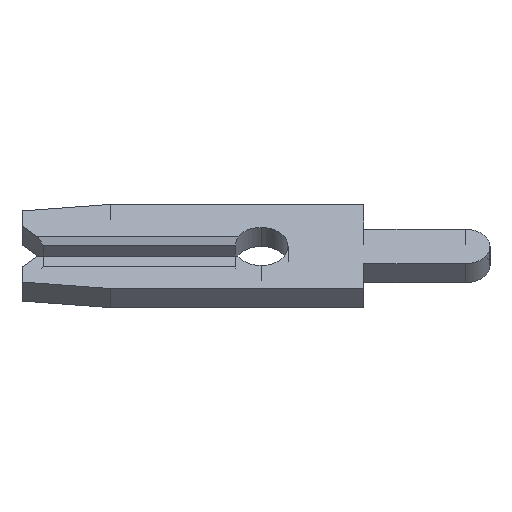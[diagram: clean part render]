
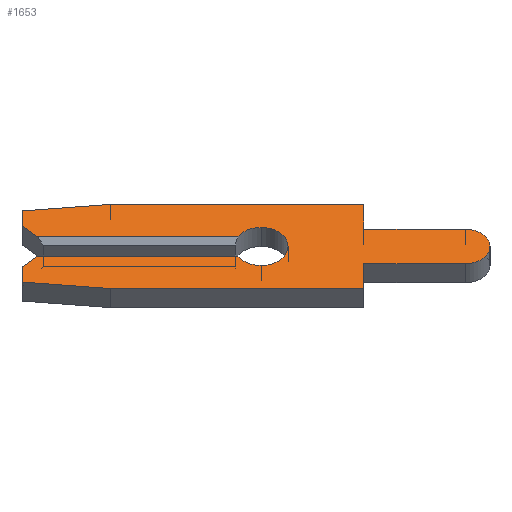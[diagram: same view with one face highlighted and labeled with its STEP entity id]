
A CAD part, left-side view. The second image highlights one B-rep face of the part: STEP entity #1653.
In plain terms, the highlighted face is planar.
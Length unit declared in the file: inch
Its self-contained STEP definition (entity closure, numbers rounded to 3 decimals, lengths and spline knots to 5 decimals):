
#2 = LINE ( 'NONE', #1609, #280 ) ;
#39 = EDGE_CURVE ( 'NONE', #1831, #1373, #1996, .T. ) ;
#45 = CARTESIAN_POINT ( 'NONE',  ( -0.013, 0., 0. ) ) ;
#47 = AXIS2_PLACEMENT_3D ( 'NONE', #45, #1066, #555 ) ;
#59 = VERTEX_POINT ( 'NONE', #773 ) ;
#92 = DIRECTION ( 'NONE',  ( 0., 0., -1. ) ) ;
#144 = AXIS2_PLACEMENT_3D ( 'NONE', #2043, #637, #298 ) ;
#159 = LINE ( 'NONE', #165, #1851 ) ;
#165 = CARTESIAN_POINT ( 'NONE',  ( -0.013, 0., -0.013 ) ) ;
#181 = VECTOR ( 'NONE', #1520, 39.37008 ) ;
#214 = AXIS2_PLACEMENT_3D ( 'NONE', #967, #972, #92 ) ;
#235 = EDGE_CURVE ( 'NONE', #1225, #517, #470, .T. ) ;
#260 = EDGE_CURVE ( 'NONE', #429, #533, #822, .T. ) ;
#280 = VECTOR ( 'NONE', #522, 39.37008 ) ;
#284 = CARTESIAN_POINT ( 'NONE',  ( -0.013, 0.2105, -0.0075 ) ) ;
#298 = DIRECTION ( 'NONE',  ( 0., 0., 1. ) ) ;
#301 = DIRECTION ( 'NONE',  ( 0., -1., 0. ) ) ;
#304 = VECTOR ( 'NONE', #2030, 39.37008 ) ;
#310 = ORIENTED_EDGE ( 'NONE', *, *, #260, .F. ) ;
#320 = CARTESIAN_POINT ( 'NONE',  ( -0.013, -0.099, -0.0235 ) ) ;
#329 = DIRECTION ( 'NONE',  ( -1., 0., 0. ) ) ;
#363 = EDGE_LOOP ( 'NONE', ( #1891, #2097, #483, #1398, #2093, #1008, #310, #1164, #1165, #1223, #1648, #1357, #1426, #921, #996, #947, #1850, #514 ) ) ;
#373 = CARTESIAN_POINT ( 'NONE',  ( -0.013, -0.099, 0.0235 ) ) ;
#401 = CARTESIAN_POINT ( 'NONE',  ( -0.013, -0.1975, -0.0235 ) ) ;
#408 = EDGE_CURVE ( 'NONE', #539, #59, #1124, .T. ) ;
#429 = VERTEX_POINT ( 'NONE', #2178 ) ;
#450 = DIRECTION ( 'NONE',  ( 0., 0.707, 0.707 ) ) ;
#460 = CARTESIAN_POINT ( 'NONE',  ( -0.013, -0.099, 0.0575 ) ) ;
#470 = LINE ( 'NONE', #995, #181 ) ;
#482 = DIRECTION ( 'NONE',  ( 0., 0., -1. ) ) ;
#483 = ORIENTED_EDGE ( 'NONE', *, *, #999, .F. ) ;
#514 = ORIENTED_EDGE ( 'NONE', *, *, #1443, .F. ) ;
#517 = VERTEX_POINT ( 'NONE', #320 ) ;
#522 = DIRECTION ( 'NONE',  ( 0., 0.995, 0.105 ) ) ;
#533 = VERTEX_POINT ( 'NONE', #1727 ) ;
#534 = CARTESIAN_POINT ( 'NONE',  ( -0.013, 0., 0. ) ) ;
#539 = VERTEX_POINT ( 'NONE', #1713 ) ;
#555 = DIRECTION ( 'NONE',  ( 0., 0., -1. ) ) ;
#559 = CARTESIAN_POINT ( 'NONE',  ( -0.013, 0.02252, -0.013 ) ) ;
#582 = LINE ( 'NONE', #460, #304 ) ;
#597 = VERTEX_POINT ( 'NONE', #1564 ) ;
#603 = VECTOR ( 'NONE', #1632, 39.37008 ) ;
#611 = DIRECTION ( 'NONE',  ( 0., 0., 1. ) ) ;
#615 = CARTESIAN_POINT ( 'NONE',  ( -0.013, 0.231, 0.028 ) ) ;
#637 = DIRECTION ( 'NONE',  ( 1., 0., 0. ) ) ;
#658 = AXIS2_PLACEMENT_3D ( 'NONE', #534, #1763, #1244 ) ;
#663 = LINE ( 'NONE', #1909, #1898 ) ;
#672 = VECTOR ( 'NONE', #1311, 39.37008 ) ;
#689 = DIRECTION ( 'NONE',  ( 0., -1., 0. ) ) ;
#695 = EDGE_CURVE ( 'NONE', #1313, #1865, #1209, .T. ) ;
#726 = EDGE_CURVE ( 'NONE', #1373, #539, #663, .T. ) ;
#771 = EDGE_CURVE ( 'NONE', #1715, #1313, #159, .T. ) ;
#773 = CARTESIAN_POINT ( 'NONE',  ( -0.013, -0.099, 0.0575 ) ) ;
#777 = VECTOR ( 'NONE', #1525, 39.37008 ) ;
#780 = VERTEX_POINT ( 'NONE', #885 ) ;
#788 = VERTEX_POINT ( 'NONE', #373 ) ;
#796 = CARTESIAN_POINT ( 'NONE',  ( -0.013, 0.231, 0.04857 ) ) ;
#806 = EDGE_CURVE ( 'NONE', #2084, #429, #2, .T. ) ;
#819 = LINE ( 'NONE', #1447, #603 ) ;
#822 = LINE ( 'NONE', #981, #1439 ) ;
#840 = EDGE_CURVE ( 'NONE', #1030, #2114, #1267, .T. ) ;
#877 = VECTOR ( 'NONE', #689, 39.37008 ) ;
#885 = CARTESIAN_POINT ( 'NONE',  ( -0.013, -0.099, -0.0575 ) ) ;
#921 = ORIENTED_EDGE ( 'NONE', *, *, #1967, .F. ) ;
#935 = VECTOR ( 'NONE', #611, 39.37008 ) ;
#947 = ORIENTED_EDGE ( 'NONE', *, *, #726, .F. ) ;
#960 = EDGE_CURVE ( 'NONE', #597, #2114, #963, .T. ) ;
#963 = LINE ( 'NONE', #1615, #1561 ) ;
#967 = CARTESIAN_POINT ( 'NONE',  ( -0.013, 0., 0. ) ) ;
#972 = DIRECTION ( 'NONE',  ( 1., 0., 0. ) ) ;
#975 = VERTEX_POINT ( 'NONE', #1780 ) ;
#981 = CARTESIAN_POINT ( 'NONE',  ( -0.013, 0.231, -0.028 ) ) ;
#987 = CARTESIAN_POINT ( 'NONE',  ( -0.013, 0.146, -0.0575 ) ) ;
#990 = LINE ( 'NONE', #2053, #877 ) ;
#995 = CARTESIAN_POINT ( 'NONE',  ( -0.013, -0.099, -0.0235 ) ) ;
#996 = ORIENTED_EDGE ( 'NONE', *, *, #408, .F. ) ;
#999 = EDGE_CURVE ( 'NONE', #1865, #1030, #1690, .T. ) ;
#1008 = ORIENTED_EDGE ( 'NONE', *, *, #1914, .F. ) ;
#1030 = VERTEX_POINT ( 'NONE', #1217 ) ;
#1050 = LINE ( 'NONE', #284, #777 ) ;
#1066 = DIRECTION ( 'NONE',  ( -1., 0., 0. ) ) ;
#1124 = LINE ( 'NONE', #1337, #1657 ) ;
#1143 = VECTOR ( 'NONE', #450, 39.37008 ) ;
#1155 = AXIS2_PLACEMENT_3D ( 'NONE', #1906, #329, #482 ) ;
#1164 = ORIENTED_EDGE ( 'NONE', *, *, #806, .F. ) ;
#1165 = ORIENTED_EDGE ( 'NONE', *, *, #1262, .F. ) ;
#1209 = CIRCLE ( 'NONE', #1155, 0.026 ) ;
#1217 = CARTESIAN_POINT ( 'NONE',  ( -0.013, 0., 0.026 ) ) ;
#1223 = ORIENTED_EDGE ( 'NONE', *, *, #1481, .F. ) ;
#1225 = VERTEX_POINT ( 'NONE', #401 ) ;
#1244 = DIRECTION ( 'NONE',  ( 0., 0., -1. ) ) ;
#1262 = EDGE_CURVE ( 'NONE', #780, #2084, #819, .T. ) ;
#1267 = CIRCLE ( 'NONE', #658, 0.026 ) ;
#1311 = DIRECTION ( 'NONE',  ( 0., 0., -1. ) ) ;
#1313 = VERTEX_POINT ( 'NONE', #559 ) ;
#1337 = CARTESIAN_POINT ( 'NONE',  ( -0.013, 0.146, 0.0575 ) ) ;
#1354 = DIRECTION ( 'NONE',  ( 0., 0., 1. ) ) ;
#1357 = ORIENTED_EDGE ( 'NONE', *, *, #1940, .F. ) ;
#1373 = VERTEX_POINT ( 'NONE', #796 ) ;
#1382 = DIRECTION ( 'NONE',  ( 0., -0.995, 0.105 ) ) ;
#1398 = ORIENTED_EDGE ( 'NONE', *, *, #695, .F. ) ;
#1426 = ORIENTED_EDGE ( 'NONE', *, *, #2123, .F. ) ;
#1439 = VECTOR ( 'NONE', #1354, 39.37008 ) ;
#1443 = EDGE_CURVE ( 'NONE', #597, #1831, #2069, .T. ) ;
#1447 = CARTESIAN_POINT ( 'NONE',  ( -0.013, 0.146, -0.0575 ) ) ;
#1470 = CIRCLE ( 'NONE', #144, 0.0235 ) ;
#1481 = EDGE_CURVE ( 'NONE', #517, #780, #1738, .T. ) ;
#1486 = CARTESIAN_POINT ( 'NONE',  ( -0.013, 0.216, -0.013 ) ) ;
#1520 = DIRECTION ( 'NONE',  ( 0., 1., 0. ) ) ;
#1525 = DIRECTION ( 'NONE',  ( 0., -0.707, 0.707 ) ) ;
#1545 = CARTESIAN_POINT ( 'NONE',  ( -0.013, 0.02252, 0.013 ) ) ;
#1554 = CARTESIAN_POINT ( 'NONE',  ( -0.013, 0.231, 0.028 ) ) ;
#1561 = VECTOR ( 'NONE', #1587, 39.37008 ) ;
#1564 = CARTESIAN_POINT ( 'NONE',  ( -0.013, 0.216, 0.013 ) ) ;
#1581 = DIRECTION ( 'NONE',  ( 0., -1., 0. ) ) ;
#1587 = DIRECTION ( 'NONE',  ( 0., -1., 0. ) ) ;
#1609 = CARTESIAN_POINT ( 'NONE',  ( -0.013, 0.231, -0.04857 ) ) ;
#1615 = CARTESIAN_POINT ( 'NONE',  ( -0.013, 0.231, 0.013 ) ) ;
#1632 = DIRECTION ( 'NONE',  ( 0., 1., 0. ) ) ;
#1648 = ORIENTED_EDGE ( 'NONE', *, *, #235, .F. ) ;
#1653 = ADVANCED_FACE ( 'NONE', ( #1669 ), #2003, .F. ) ;
#1657 = VECTOR ( 'NONE', #301, 39.37008 ) ;
#1661 = CARTESIAN_POINT ( 'NONE',  ( -0.013, -0.099, -0.0575 ) ) ;
#1669 = FACE_OUTER_BOUND ( 'NONE', #363, .T. ) ;
#1675 = CARTESIAN_POINT ( 'NONE',  ( -0.013, 0., -0.026 ) ) ;
#1690 = CIRCLE ( 'NONE', #47, 0.026 ) ;
#1713 = CARTESIAN_POINT ( 'NONE',  ( -0.013, 0.146, 0.0575 ) ) ;
#1715 = VERTEX_POINT ( 'NONE', #1486 ) ;
#1727 = CARTESIAN_POINT ( 'NONE',  ( -0.013, 0.231, -0.028 ) ) ;
#1738 = LINE ( 'NONE', #1661, #672 ) ;
#1763 = DIRECTION ( 'NONE',  ( -1., 0., 0. ) ) ;
#1780 = CARTESIAN_POINT ( 'NONE',  ( -0.013, -0.1975, 0.0235 ) ) ;
#1831 = VERTEX_POINT ( 'NONE', #1554 ) ;
#1850 = ORIENTED_EDGE ( 'NONE', *, *, #39, .F. ) ;
#1851 = VECTOR ( 'NONE', #1581, 39.37008 ) ;
#1865 = VERTEX_POINT ( 'NONE', #1675 ) ;
#1891 = ORIENTED_EDGE ( 'NONE', *, *, #960, .T. ) ;
#1898 = VECTOR ( 'NONE', #1382, 39.37008 ) ;
#1906 = CARTESIAN_POINT ( 'NONE',  ( -0.013, 0., 0. ) ) ;
#1909 = CARTESIAN_POINT ( 'NONE',  ( -0.013, 0.231, 0.04857 ) ) ;
#1914 = EDGE_CURVE ( 'NONE', #533, #1715, #1050, .T. ) ;
#1940 = EDGE_CURVE ( 'NONE', #975, #1225, #1470, .T. ) ;
#1967 = EDGE_CURVE ( 'NONE', #59, #788, #582, .T. ) ;
#1996 = LINE ( 'NONE', #615, #935 ) ;
#2003 = PLANE ( 'NONE',  #214 ) ;
#2030 = DIRECTION ( 'NONE',  ( 0., 0., -1. ) ) ;
#2043 = CARTESIAN_POINT ( 'NONE',  ( -0.013, -0.1975, 0. ) ) ;
#2053 = CARTESIAN_POINT ( 'NONE',  ( -0.013, -0.099, 0.0235 ) ) ;
#2069 = LINE ( 'NONE', #2175, #1143 ) ;
#2084 = VERTEX_POINT ( 'NONE', #987 ) ;
#2093 = ORIENTED_EDGE ( 'NONE', *, *, #771, .F. ) ;
#2097 = ORIENTED_EDGE ( 'NONE', *, *, #840, .F. ) ;
#2114 = VERTEX_POINT ( 'NONE', #1545 ) ;
#2123 = EDGE_CURVE ( 'NONE', #788, #975, #990, .T. ) ;
#2175 = CARTESIAN_POINT ( 'NONE',  ( -0.013, 0.2105, 0.0075 ) ) ;
#2178 = CARTESIAN_POINT ( 'NONE',  ( -0.013, 0.231, -0.04857 ) ) ;
